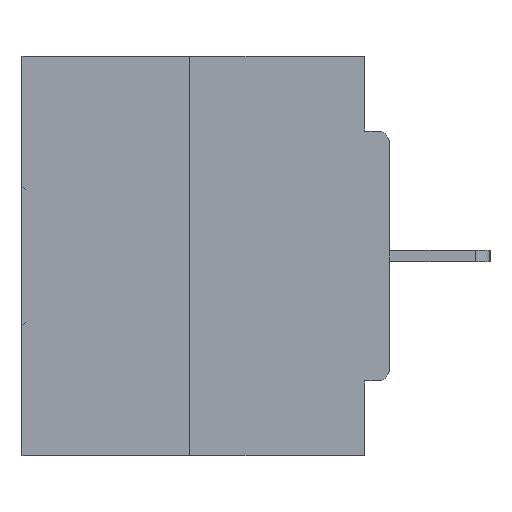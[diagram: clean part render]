
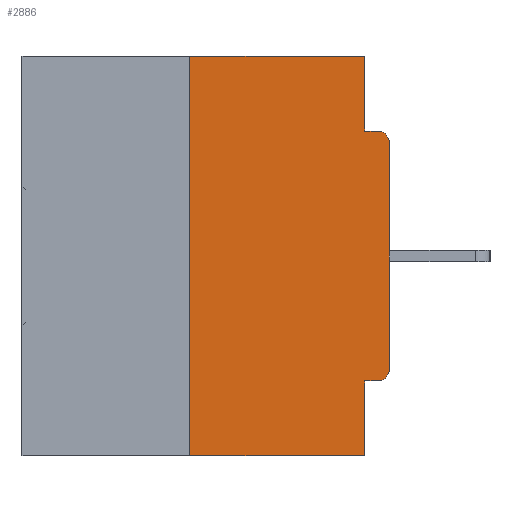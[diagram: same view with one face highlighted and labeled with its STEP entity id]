
A CAD part, left-side view. The second image highlights one B-rep face of the part: STEP entity #2886.
In plain terms, the highlighted planar face has unit normal (-1, 0, 0).
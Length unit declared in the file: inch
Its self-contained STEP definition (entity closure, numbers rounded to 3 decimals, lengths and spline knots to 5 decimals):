
#123 = AXIS2_PLACEMENT_3D ( 'NONE', #15999, #18986, #1142 ) ;
#150 = VERTEX_POINT ( 'NONE', #35492 ) ;
#1142 = DIRECTION ( 'NONE',  ( 0., 0., -1. ) ) ;
#1582 = CARTESIAN_POINT ( 'NONE',  ( 0., 0.25, 0. ) ) ;
#2261 = VECTOR ( 'NONE', #6133, 39.37008 ) ;
#2537 = CARTESIAN_POINT ( 'NONE',  ( 0., 0., -0.1085 ) ) ;
#2886 = ADVANCED_FACE ( 'NONE', ( #18639 ), #33303, .F. ) ;
#3036 = LINE ( 'NONE', #1582, #9080 ) ;
#3170 = ORIENTED_EDGE ( 'NONE', *, *, #20889, .F. ) ;
#3238 = VECTOR ( 'NONE', #15288, 39.37008 ) ;
#3355 = CARTESIAN_POINT ( 'NONE',  ( 0., 0.031, -0.4065 ) ) ;
#3529 = VERTEX_POINT ( 'NONE', #36258 ) ;
#3644 = DIRECTION ( 'NONE',  ( -1., 0., 0. ) ) ;
#4177 = VERTEX_POINT ( 'NONE', #33341 ) ;
#4282 = VERTEX_POINT ( 'NONE', #36824 ) ;
#4423 = LINE ( 'NONE', #7299, #33673 ) ;
#5291 = CARTESIAN_POINT ( 'NONE',  ( 0., 0., -0.4065 ) ) ;
#5474 = EDGE_CURVE ( 'NONE', #4282, #150, #36011, .T. ) ;
#5711 = ORIENTED_EDGE ( 'NONE', *, *, #37262, .F. ) ;
#5717 = CARTESIAN_POINT ( 'NONE',  ( 0., 0.015, -0.1085 ) ) ;
#5765 = ORIENTED_EDGE ( 'NONE', *, *, #5474, .F. ) ;
#5918 = VERTEX_POINT ( 'NONE', #10329 ) ;
#6133 = DIRECTION ( 'NONE',  ( 0., 0., -1. ) ) ;
#6137 = ORIENTED_EDGE ( 'NONE', *, *, #36094, .T. ) ;
#6858 = VECTOR ( 'NONE', #25853, 39.37008 ) ;
#7299 = CARTESIAN_POINT ( 'NONE',  ( 0., 0.46, -0.5 ) ) ;
#7553 = ORIENTED_EDGE ( 'NONE', *, *, #11841, .T. ) ;
#8291 = DIRECTION ( 'NONE',  ( 0., 1., 0. ) ) ;
#8378 = VERTEX_POINT ( 'NONE', #16029 ) ;
#8691 = DIRECTION ( 'NONE',  ( 0., 0., -1. ) ) ;
#9080 = VECTOR ( 'NONE', #25314, 39.37008 ) ;
#10130 = VECTOR ( 'NONE', #12447, 39.37008 ) ;
#10293 = DIRECTION ( 'NONE',  ( 0., -1., 0. ) ) ;
#10329 = CARTESIAN_POINT ( 'NONE',  ( 0., 0.015, -0.4065 ) ) ;
#11751 = VERTEX_POINT ( 'NONE', #2537 ) ;
#11841 = EDGE_CURVE ( 'NONE', #8378, #11751, #33343, .T. ) ;
#11847 = CARTESIAN_POINT ( 'NONE',  ( 0., 0.031, 0. ) ) ;
#12420 = CARTESIAN_POINT ( 'NONE',  ( 0., 0., -0.0935 ) ) ;
#12447 = DIRECTION ( 'NONE',  ( 0., 0., 1. ) ) ;
#13479 = ORIENTED_EDGE ( 'NONE', *, *, #16274, .F. ) ;
#13556 = DIRECTION ( 'NONE',  ( 0., 0., -1. ) ) ;
#15081 = VERTEX_POINT ( 'NONE', #3355 ) ;
#15288 = DIRECTION ( 'NONE',  ( 0., -1., 0. ) ) ;
#15999 = CARTESIAN_POINT ( 'NONE',  ( 0., 0.46, 0. ) ) ;
#16029 = CARTESIAN_POINT ( 'NONE',  ( 0., 0., -0.3915 ) ) ;
#16274 = EDGE_CURVE ( 'NONE', #150, #19412, #18100, .T. ) ;
#16384 = EDGE_CURVE ( 'NONE', #5918, #8378, #22165, .T. ) ;
#17772 = ORIENTED_EDGE ( 'NONE', *, *, #31138, .F. ) ;
#18100 = LINE ( 'NONE', #11847, #2261 ) ;
#18639 = FACE_OUTER_BOUND ( 'NONE', #18763, .T. ) ;
#18763 = EDGE_LOOP ( 'NONE', ( #5765, #17772, #32996, #3170, #36055, #28382, #7553, #6137, #5711, #13479 ) ) ;
#18986 = DIRECTION ( 'NONE',  ( 1., 0., 0. ) ) ;
#19412 = VERTEX_POINT ( 'NONE', #22631 ) ;
#20834 = EDGE_CURVE ( 'NONE', #3529, #36202, #4423, .T. ) ;
#20889 = EDGE_CURVE ( 'NONE', #15081, #36202, #26045, .T. ) ;
#21375 = CARTESIAN_POINT ( 'NONE',  ( 0., 0.015, -0.3915 ) ) ;
#21659 = EDGE_CURVE ( 'NONE', #5918, #15081, #35415, .T. ) ;
#22165 = CIRCLE ( 'NONE', #30621, 0.015 ) ;
#22631 = CARTESIAN_POINT ( 'NONE',  ( 0., 0.031, -0.0935 ) ) ;
#24272 = DIRECTION ( 'NONE',  ( 0., 0., -1. ) ) ;
#25314 = DIRECTION ( 'NONE',  ( 0., 0., 1. ) ) ;
#25853 = DIRECTION ( 'NONE',  ( 0., -1., 0. ) ) ;
#26045 = LINE ( 'NONE', #28056, #31887 ) ;
#26261 = DIRECTION ( 'NONE',  ( -1., 0., 0. ) ) ;
#26641 = CARTESIAN_POINT ( 'NONE',  ( 0., 0.031, -0.5 ) ) ;
#28056 = CARTESIAN_POINT ( 'NONE',  ( 0., 0.031, -0.5 ) ) ;
#28382 = ORIENTED_EDGE ( 'NONE', *, *, #16384, .T. ) ;
#29193 = CIRCLE ( 'NONE', #30878, 0.015 ) ;
#29422 = LINE ( 'NONE', #12420, #3238 ) ;
#30621 = AXIS2_PLACEMENT_3D ( 'NONE', #21375, #3644, #24272 ) ;
#30878 = AXIS2_PLACEMENT_3D ( 'NONE', #5717, #26261, #8691 ) ;
#31138 = EDGE_CURVE ( 'NONE', #3529, #4282, #3036, .T. ) ;
#31887 = VECTOR ( 'NONE', #13556, 39.37008 ) ;
#32996 = ORIENTED_EDGE ( 'NONE', *, *, #20834, .T. ) ;
#33303 = PLANE ( 'NONE',  #123 ) ;
#33341 = CARTESIAN_POINT ( 'NONE',  ( 0., 0.015, -0.0935 ) ) ;
#33343 = LINE ( 'NONE', #35009, #10130 ) ;
#33673 = VECTOR ( 'NONE', #10293, 39.37008 ) ;
#34526 = VECTOR ( 'NONE', #8291, 39.37008 ) ;
#35009 = CARTESIAN_POINT ( 'NONE',  ( 0., 0., 0. ) ) ;
#35415 = LINE ( 'NONE', #5291, #34526 ) ;
#35492 = CARTESIAN_POINT ( 'NONE',  ( 0., 0.031, 0. ) ) ;
#36011 = LINE ( 'NONE', #37368, #6858 ) ;
#36055 = ORIENTED_EDGE ( 'NONE', *, *, #21659, .F. ) ;
#36094 = EDGE_CURVE ( 'NONE', #11751, #4177, #29193, .T. ) ;
#36202 = VERTEX_POINT ( 'NONE', #26641 ) ;
#36258 = CARTESIAN_POINT ( 'NONE',  ( 0., 0.25, -0.5 ) ) ;
#36824 = CARTESIAN_POINT ( 'NONE',  ( 0., 0.25, 0. ) ) ;
#37262 = EDGE_CURVE ( 'NONE', #19412, #4177, #29422, .T. ) ;
#37368 = CARTESIAN_POINT ( 'NONE',  ( 0., 0.46, 0. ) ) ;
